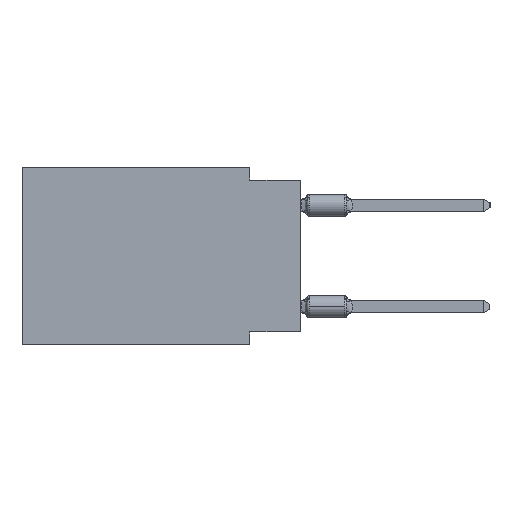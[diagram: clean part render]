
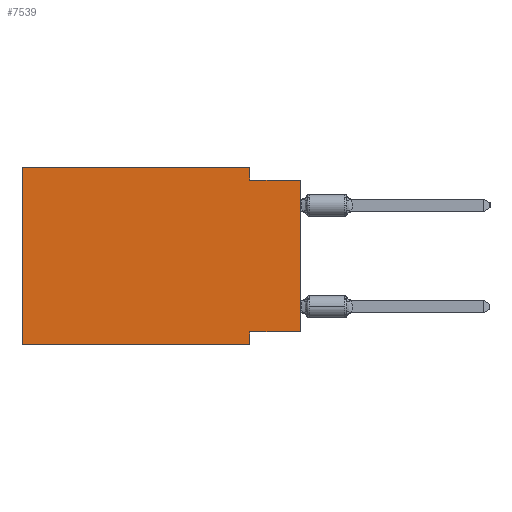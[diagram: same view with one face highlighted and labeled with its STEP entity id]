
A CAD part, left-side view. The second image highlights one B-rep face of the part: STEP entity #7539.
In plain terms, the highlighted planar face has unit normal (-1, 0, 0).
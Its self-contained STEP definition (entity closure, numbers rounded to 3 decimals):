
#32 = VECTOR ( 'NONE', #15723, 1000. ) ;
#227 = ORIENTED_EDGE ( 'NONE', *, *, #8168, .F. ) ;
#556 = CARTESIAN_POINT ( 'NONE',  ( 0., 2.54, 0. ) ) ;
#622 = DIRECTION ( 'NONE',  ( 0., 0., -1. ) ) ;
#1128 = ORIENTED_EDGE ( 'NONE', *, *, #3266, .F. ) ;
#1363 = CARTESIAN_POINT ( 'NONE',  ( 0., 0., -8.255 ) ) ;
#1424 = CARTESIAN_POINT ( 'NONE',  ( 0., 13.97, 0. ) ) ;
#1591 = CARTESIAN_POINT ( 'NONE',  ( 0., 0., 0. ) ) ;
#1662 = PLANE ( 'NONE',  #19145 ) ;
#2187 = CARTESIAN_POINT ( 'NONE',  ( 0., 13.97, 0. ) ) ;
#2454 = CARTESIAN_POINT ( 'NONE',  ( 0., 2.54, -8.89 ) ) ;
#2526 = VECTOR ( 'NONE', #21061, 1000. ) ;
#2615 = VECTOR ( 'NONE', #3323, 1000. ) ;
#3006 = LINE ( 'NONE', #4527, #2526 ) ;
#3198 = LINE ( 'NONE', #1363, #6638 ) ;
#3266 = EDGE_CURVE ( 'NONE', #14390, #4083, #3198, .T. ) ;
#3323 = DIRECTION ( 'NONE',  ( 0., 0., 1. ) ) ;
#4022 = VERTEX_POINT ( 'NONE', #6194 ) ;
#4083 = VERTEX_POINT ( 'NONE', #16210 ) ;
#4242 = EDGE_CURVE ( 'NONE', #4083, #18313, #20613, .T. ) ;
#4328 = VERTEX_POINT ( 'NONE', #20938 ) ;
#4527 = CARTESIAN_POINT ( 'NONE',  ( 0., 13.97, 0. ) ) ;
#4548 = CARTESIAN_POINT ( 'NONE',  ( 0., 2.54, -8.89 ) ) ;
#6194 = CARTESIAN_POINT ( 'NONE',  ( 0., 13.97, -8.89 ) ) ;
#6451 = ORIENTED_EDGE ( 'NONE', *, *, #11116, .F. ) ;
#6638 = VECTOR ( 'NONE', #19828, 1000. ) ;
#7539 = ADVANCED_FACE ( 'NONE', ( #14909 ), #1662, .F. ) ;
#7916 = ORIENTED_EDGE ( 'NONE', *, *, #4242, .F. ) ;
#8168 = EDGE_CURVE ( 'NONE', #4022, #9309, #3006, .T. ) ;
#8284 = CARTESIAN_POINT ( 'NONE',  ( 0., 13.97, 0. ) ) ;
#8838 = ORIENTED_EDGE ( 'NONE', *, *, #15850, .F. ) ;
#8912 = EDGE_LOOP ( 'NONE', ( #17980, #6451, #15709, #8838, #227, #15626, #7916, #1128 ) ) ;
#9298 = CARTESIAN_POINT ( 'NONE',  ( 0., 2.54, 0. ) ) ;
#9304 = VECTOR ( 'NONE', #14599, 1000. ) ;
#9309 = VERTEX_POINT ( 'NONE', #1424 ) ;
#9963 = VERTEX_POINT ( 'NONE', #9298 ) ;
#10738 = VECTOR ( 'NONE', #622, 1000. ) ;
#11058 = VERTEX_POINT ( 'NONE', #20509 ) ;
#11116 = EDGE_CURVE ( 'NONE', #4328, #11058, #17260, .T. ) ;
#11973 = DIRECTION ( 'NONE',  ( 0., -1., 0. ) ) ;
#12852 = DIRECTION ( 'NONE',  ( 0., 0., -1. ) ) ;
#12858 = EDGE_CURVE ( 'NONE', #9963, #4328, #16958, .T. ) ;
#12864 = CARTESIAN_POINT ( 'NONE',  ( 0., 13.97, -8.89 ) ) ;
#13797 = LINE ( 'NONE', #2187, #14538 ) ;
#14390 = VERTEX_POINT ( 'NONE', #15784 ) ;
#14538 = VECTOR ( 'NONE', #11973, 1000. ) ;
#14599 = DIRECTION ( 'NONE',  ( 0., -1., 0. ) ) ;
#14649 = VECTOR ( 'NONE', #17062, 1000. ) ;
#14706 = LINE ( 'NONE', #12864, #9304 ) ;
#14729 = LINE ( 'NONE', #1591, #2615 ) ;
#14909 = FACE_OUTER_BOUND ( 'NONE', #8912, .T. ) ;
#15310 = EDGE_CURVE ( 'NONE', #4022, #18313, #14706, .T. ) ;
#15626 = ORIENTED_EDGE ( 'NONE', *, *, #15310, .T. ) ;
#15709 = ORIENTED_EDGE ( 'NONE', *, *, #12858, .F. ) ;
#15723 = DIRECTION ( 'NONE',  ( 0., -1., 0. ) ) ;
#15784 = CARTESIAN_POINT ( 'NONE',  ( 0., 0., -8.255 ) ) ;
#15850 = EDGE_CURVE ( 'NONE', #9309, #9963, #13797, .T. ) ;
#16210 = CARTESIAN_POINT ( 'NONE',  ( 0., 2.54, -8.255 ) ) ;
#16958 = LINE ( 'NONE', #556, #14649 ) ;
#17062 = DIRECTION ( 'NONE',  ( 0., 0., -1. ) ) ;
#17260 = LINE ( 'NONE', #18988, #32 ) ;
#17980 = ORIENTED_EDGE ( 'NONE', *, *, #18814, .T. ) ;
#18185 = DIRECTION ( 'NONE',  ( 1., 0., 0. ) ) ;
#18313 = VERTEX_POINT ( 'NONE', #4548 ) ;
#18814 = EDGE_CURVE ( 'NONE', #14390, #11058, #14729, .T. ) ;
#18988 = CARTESIAN_POINT ( 'NONE',  ( 0., 0., -0.635 ) ) ;
#19145 = AXIS2_PLACEMENT_3D ( 'NONE', #8284, #18185, #12852 ) ;
#19828 = DIRECTION ( 'NONE',  ( 0., 1., 0. ) ) ;
#20509 = CARTESIAN_POINT ( 'NONE',  ( 0., 0., -0.635 ) ) ;
#20613 = LINE ( 'NONE', #2454, #10738 ) ;
#20938 = CARTESIAN_POINT ( 'NONE',  ( 0., 2.54, -0.635 ) ) ;
#21061 = DIRECTION ( 'NONE',  ( 0., 0., 1. ) ) ;
